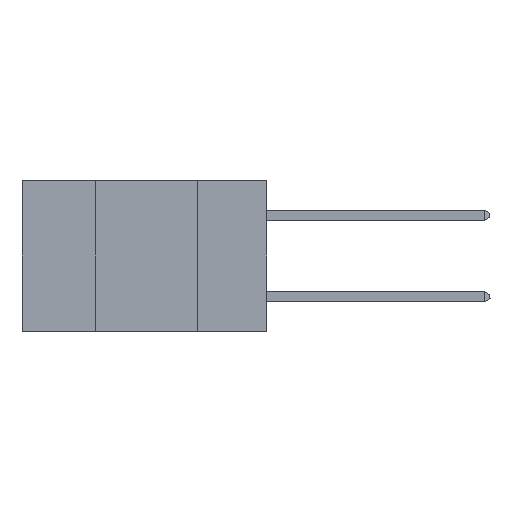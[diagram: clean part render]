
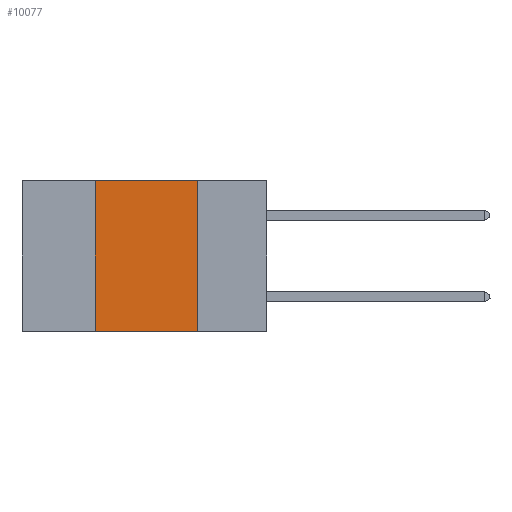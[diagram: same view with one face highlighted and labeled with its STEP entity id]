
A CAD part, left-side view. The second image highlights one B-rep face of the part: STEP entity #10077.
In plain terms, the highlighted planar face has unit normal (-1, 0, 0).
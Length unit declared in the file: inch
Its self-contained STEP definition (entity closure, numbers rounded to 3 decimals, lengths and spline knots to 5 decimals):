
#822 = VECTOR ( 'NONE', #2524, 39.37008 ) ;
#1283 = DIRECTION ( 'NONE',  ( 0., 0., -1. ) ) ;
#1342 = DIRECTION ( 'NONE',  ( 1., 0., 0. ) ) ;
#1863 = EDGE_CURVE ( 'NONE', #9056, #8572, #10759, .T. ) ;
#2524 = DIRECTION ( 'NONE',  ( 0., -1., 0. ) ) ;
#3006 = CARTESIAN_POINT ( 'NONE',  ( 0., 0.42, -0.37 ) ) ;
#4471 = VECTOR ( 'NONE', #17153, 39.37008 ) ;
#4680 = VECTOR ( 'NONE', #5944, 39.37008 ) ;
#5343 = CARTESIAN_POINT ( 'NONE',  ( 0., 0.17, 0. ) ) ;
#5944 = DIRECTION ( 'NONE',  ( 0., -1., 0. ) ) ;
#6990 = AXIS2_PLACEMENT_3D ( 'NONE', #9395, #1342, #1283 ) ;
#7045 = CARTESIAN_POINT ( 'NONE',  ( 0., 0.17, -0.37 ) ) ;
#8312 = PLANE ( 'NONE',  #6990 ) ;
#8572 = VERTEX_POINT ( 'NONE', #11401 ) ;
#8599 = ORIENTED_EDGE ( 'NONE', *, *, #1863, .F. ) ;
#9056 = VERTEX_POINT ( 'NONE', #15228 ) ;
#9237 = ORIENTED_EDGE ( 'NONE', *, *, #9613, .F. ) ;
#9277 = CARTESIAN_POINT ( 'NONE',  ( 0., 0.6, 0. ) ) ;
#9395 = CARTESIAN_POINT ( 'NONE',  ( 0., 0.6, 0. ) ) ;
#9613 = EDGE_CURVE ( 'NONE', #11756, #9056, #10395, .T. ) ;
#9652 = CARTESIAN_POINT ( 'NONE',  ( 0., 0.42, 0. ) ) ;
#9895 = EDGE_LOOP ( 'NONE', ( #15681, #8599, #9237, #13937 ) ) ;
#10077 = ADVANCED_FACE ( 'NONE', ( #12045 ), #8312, .F. ) ;
#10395 = LINE ( 'NONE', #9652, #4471 ) ;
#10759 = LINE ( 'NONE', #9277, #822 ) ;
#11401 = CARTESIAN_POINT ( 'NONE',  ( 0., 0.17, 0. ) ) ;
#11756 = VERTEX_POINT ( 'NONE', #3006 ) ;
#12045 = FACE_OUTER_BOUND ( 'NONE', #9895, .T. ) ;
#12102 = DIRECTION ( 'NONE',  ( 0., 0., -1. ) ) ;
#12375 = EDGE_CURVE ( 'NONE', #11756, #17247, #14994, .T. ) ;
#13633 = VECTOR ( 'NONE', #12102, 39.37008 ) ;
#13783 = CARTESIAN_POINT ( 'NONE',  ( 0., 0.6, -0.37 ) ) ;
#13937 = ORIENTED_EDGE ( 'NONE', *, *, #12375, .T. ) ;
#14994 = LINE ( 'NONE', #13783, #4680 ) ;
#15102 = LINE ( 'NONE', #5343, #13633 ) ;
#15152 = EDGE_CURVE ( 'NONE', #8572, #17247, #15102, .T. ) ;
#15228 = CARTESIAN_POINT ( 'NONE',  ( 0., 0.42, 0. ) ) ;
#15681 = ORIENTED_EDGE ( 'NONE', *, *, #15152, .F. ) ;
#17153 = DIRECTION ( 'NONE',  ( 0., 0., 1. ) ) ;
#17247 = VERTEX_POINT ( 'NONE', #7045 ) ;
